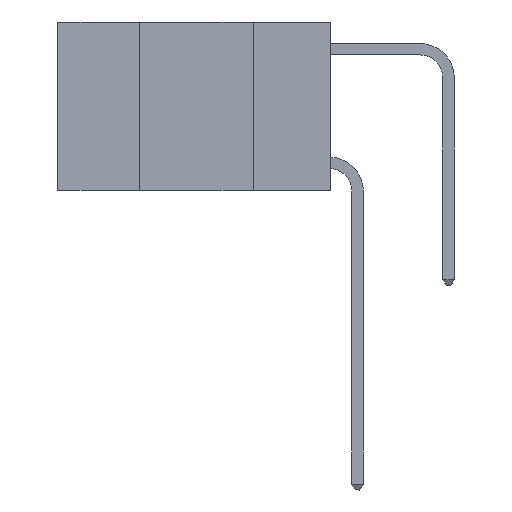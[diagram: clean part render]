
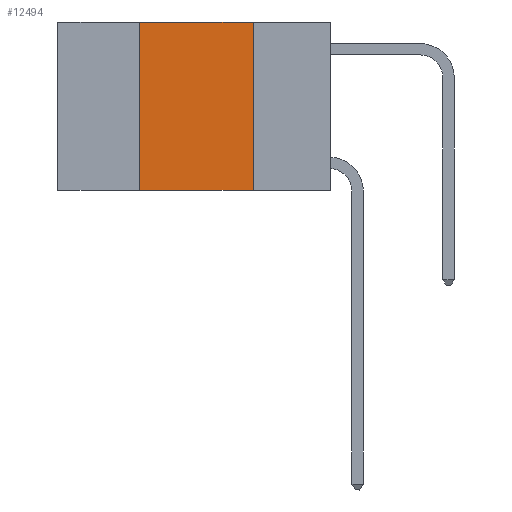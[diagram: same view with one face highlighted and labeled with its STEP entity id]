
A CAD part, left-side view. The second image highlights one B-rep face of the part: STEP entity #12494.
In plain terms, the highlighted planar face has unit normal (-1, 0, 0).
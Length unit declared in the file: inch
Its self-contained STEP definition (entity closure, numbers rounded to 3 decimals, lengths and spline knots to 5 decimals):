
#163 = VERTEX_POINT ( 'NONE', #7207 ) ;
#221 = VECTOR ( 'NONE', #15358, 39.37008 ) ;
#549 = EDGE_CURVE ( 'NONE', #18560, #16855, #11185, .T. ) ;
#970 = PLANE ( 'NONE',  #19507 ) ;
#2460 = VECTOR ( 'NONE', #4190, 39.37008 ) ;
#3822 = VECTOR ( 'NONE', #14979, 39.37008 ) ;
#4190 = DIRECTION ( 'NONE',  ( 0., 0., -1. ) ) ;
#4328 = FACE_OUTER_BOUND ( 'NONE', #9657, .T. ) ;
#7207 = CARTESIAN_POINT ( 'NONE',  ( 0., 0.42, 0. ) ) ;
#7362 = ORIENTED_EDGE ( 'NONE', *, *, #549, .F. ) ;
#8589 = LINE ( 'NONE', #12636, #221 ) ;
#8859 = VERTEX_POINT ( 'NONE', #11798 ) ;
#9657 = EDGE_LOOP ( 'NONE', ( #7362, #25267, #26578, #13400 ) ) ;
#10630 = EDGE_CURVE ( 'NONE', #8859, #16855, #25343, .T. ) ;
#11185 = LINE ( 'NONE', #12511, #2460 ) ;
#11798 = CARTESIAN_POINT ( 'NONE',  ( 0., 0.42, -0.37 ) ) ;
#12467 = CARTESIAN_POINT ( 'NONE',  ( 0., 0.17, -0.37 ) ) ;
#12494 = ADVANCED_FACE ( 'NONE', ( #4328 ), #970, .F. ) ;
#12511 = CARTESIAN_POINT ( 'NONE',  ( 0., 0.17, 0. ) ) ;
#12636 = CARTESIAN_POINT ( 'NONE',  ( 0., 0.42, 0. ) ) ;
#12768 = DIRECTION ( 'NONE',  ( 0., 0., -1. ) ) ;
#13400 = ORIENTED_EDGE ( 'NONE', *, *, #10630, .T. ) ;
#14227 = DIRECTION ( 'NONE',  ( 0., -1., 0. ) ) ;
#14979 = DIRECTION ( 'NONE',  ( 0., -1., 0. ) ) ;
#15116 = CARTESIAN_POINT ( 'NONE',  ( 0., 0.6, 0. ) ) ;
#15173 = CARTESIAN_POINT ( 'NONE',  ( 0., 0.6, 0. ) ) ;
#15358 = DIRECTION ( 'NONE',  ( 0., 0., 1. ) ) ;
#16855 = VERTEX_POINT ( 'NONE', #12467 ) ;
#18560 = VERTEX_POINT ( 'NONE', #25189 ) ;
#19507 = AXIS2_PLACEMENT_3D ( 'NONE', #15116, #23927, #12768 ) ;
#20549 = LINE ( 'NONE', #15173, #3822 ) ;
#23233 = EDGE_CURVE ( 'NONE', #163, #18560, #20549, .T. ) ;
#23927 = DIRECTION ( 'NONE',  ( 1., 0., 0. ) ) ;
#24305 = VECTOR ( 'NONE', #14227, 39.37008 ) ;
#25068 = EDGE_CURVE ( 'NONE', #8859, #163, #8589, .T. ) ;
#25189 = CARTESIAN_POINT ( 'NONE',  ( 0., 0.17, 0. ) ) ;
#25267 = ORIENTED_EDGE ( 'NONE', *, *, #23233, .F. ) ;
#25343 = LINE ( 'NONE', #25949, #24305 ) ;
#25949 = CARTESIAN_POINT ( 'NONE',  ( 0., 0.6, -0.37 ) ) ;
#26578 = ORIENTED_EDGE ( 'NONE', *, *, #25068, .F. ) ;
